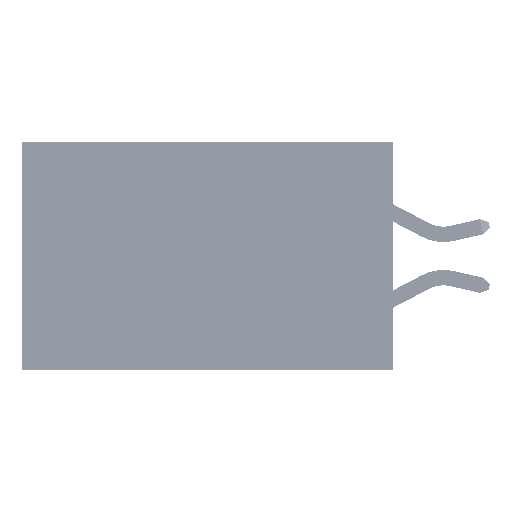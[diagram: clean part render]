
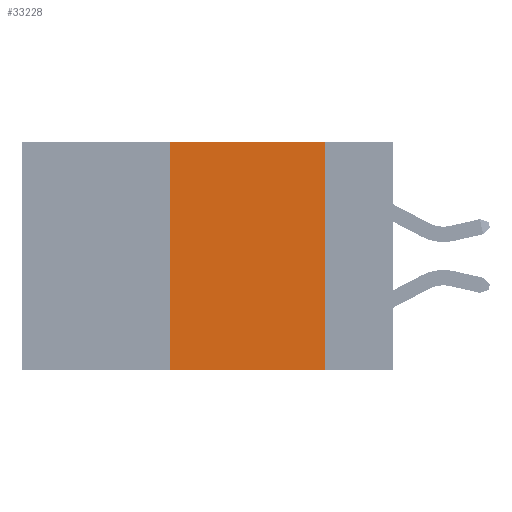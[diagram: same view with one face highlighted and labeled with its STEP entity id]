
A CAD part, left-side view. The second image highlights one B-rep face of the part: STEP entity #33228.
In plain terms, the highlighted planar face has unit normal (-1, 0, 0).
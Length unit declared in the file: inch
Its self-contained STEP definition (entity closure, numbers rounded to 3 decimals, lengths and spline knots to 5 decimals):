
#2117 = AXIS2_PLACEMENT_3D ( 'NONE', #17252, #39933, #17410 ) ;
#9109 = CARTESIAN_POINT ( 'NONE',  ( 0., 0.36, 0. ) ) ;
#9685 = EDGE_CURVE ( 'NONE', #43916, #21621, #25150, .T. ) ;
#9930 = VERTEX_POINT ( 'NONE', #31769 ) ;
#10164 = VECTOR ( 'NONE', #39330, 39.37008 ) ;
#10643 = EDGE_CURVE ( 'NONE', #9930, #29418, #12558, .T. ) ;
#11876 = DIRECTION ( 'NONE',  ( 0., -1., 0. ) ) ;
#12558 = LINE ( 'NONE', #9109, #10164 ) ;
#15010 = VECTOR ( 'NONE', #11876, 39.37008 ) ;
#15046 = VECTOR ( 'NONE', #22828, 39.37008 ) ;
#17092 = DIRECTION ( 'NONE',  ( 0., -1., 0. ) ) ;
#17252 = CARTESIAN_POINT ( 'NONE',  ( 0., 0.6, 0. ) ) ;
#17410 = DIRECTION ( 'NONE',  ( 0., 0., -1. ) ) ;
#17645 = ORIENTED_EDGE ( 'NONE', *, *, #9685, .F. ) ;
#21196 = ORIENTED_EDGE ( 'NONE', *, *, #10643, .F. ) ;
#21621 = VERTEX_POINT ( 'NONE', #38979 ) ;
#22828 = DIRECTION ( 'NONE',  ( 0., 0., -1. ) ) ;
#23236 = EDGE_LOOP ( 'NONE', ( #17645, #30087, #21196, #43482 ) ) ;
#25121 = LINE ( 'NONE', #26992, #15010 ) ;
#25150 = LINE ( 'NONE', #37649, #15046 ) ;
#26870 = EDGE_CURVE ( 'NONE', #9930, #21621, #25121, .T. ) ;
#26992 = CARTESIAN_POINT ( 'NONE',  ( 0., 0.6, -0.37 ) ) ;
#29418 = VERTEX_POINT ( 'NONE', #32333 ) ;
#30087 = ORIENTED_EDGE ( 'NONE', *, *, #36260, .F. ) ;
#30363 = LINE ( 'NONE', #46907, #39089 ) ;
#31769 = CARTESIAN_POINT ( 'NONE',  ( 0., 0.36, -0.37 ) ) ;
#32333 = CARTESIAN_POINT ( 'NONE',  ( 0., 0.36, 0. ) ) ;
#33228 = ADVANCED_FACE ( 'NONE', ( #36817 ), #36249, .F. ) ;
#36249 = PLANE ( 'NONE',  #2117 ) ;
#36260 = EDGE_CURVE ( 'NONE', #29418, #43916, #30363, .T. ) ;
#36817 = FACE_OUTER_BOUND ( 'NONE', #23236, .T. ) ;
#37649 = CARTESIAN_POINT ( 'NONE',  ( 0., 0.11, 0. ) ) ;
#38979 = CARTESIAN_POINT ( 'NONE',  ( 0., 0.11, -0.37 ) ) ;
#39089 = VECTOR ( 'NONE', #17092, 39.37008 ) ;
#39330 = DIRECTION ( 'NONE',  ( 0., 0., 1. ) ) ;
#39933 = DIRECTION ( 'NONE',  ( 1., 0., 0. ) ) ;
#42337 = CARTESIAN_POINT ( 'NONE',  ( 0., 0.11, 0. ) ) ;
#43482 = ORIENTED_EDGE ( 'NONE', *, *, #26870, .T. ) ;
#43916 = VERTEX_POINT ( 'NONE', #42337 ) ;
#46907 = CARTESIAN_POINT ( 'NONE',  ( 0., 0.6, 0. ) ) ;
